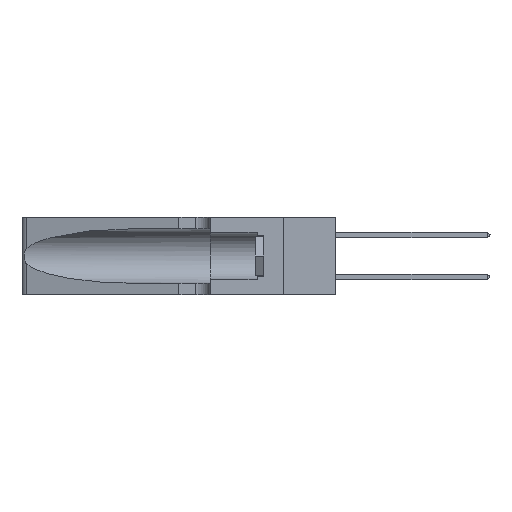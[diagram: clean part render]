
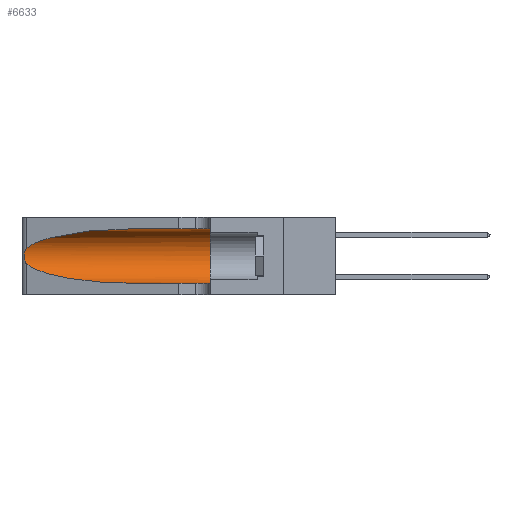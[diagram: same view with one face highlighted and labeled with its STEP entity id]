
A CAD part, left-side view. The second image highlights one B-rep face of the part: STEP entity #6633.
In plain terms, the highlighted cylindrical face has radius 3.308 mm (diameter 6.617 mm), a partial arc.
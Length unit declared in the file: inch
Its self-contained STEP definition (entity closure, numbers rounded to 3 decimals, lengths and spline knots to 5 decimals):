
#329 = CARTESIAN_POINT ( 'NONE',  ( 0.1305, 1.61858, 0.31525 ) ) ;
#985 = CARTESIAN_POINT ( 'NONE',  ( 0.25854, 1.2359, 0.20912 ) ) ;
#3016 = VERTEX_POINT ( 'NONE', #15872 ) ;
#3162 = CARTESIAN_POINT ( 'NONE',  ( 0.25487, 1.22718, 0.22369 ) ) ;
#3678 = DIRECTION ( 'NONE',  ( 0., 1., 0. ) ) ;
#3723 = CARTESIAN_POINT ( 'NONE',  ( 0.26075, 1.23896, 0.19203 ) ) ;
#4461 =( BOUNDED_CURVE ( )  B_SPLINE_CURVE ( 3, ( #12439, #17626, #32968, #30486 ),
 .UNSPECIFIED., .F., .T. ) 
 B_SPLINE_CURVE_WITH_KNOTS ( ( 4, 4 ),
 ( 1.5708, 2.84003 ),
 .UNSPECIFIED. ) 
 CURVE ( )  GEOMETRIC_REPRESENTATION_ITEM ( )  RATIONAL_B_SPLINE_CURVE ( ( 1., 0.87, 0.87, 1. ) ) 
 REPRESENTATION_ITEM ( '' )  );
#5257 = CYLINDRICAL_SURFACE ( 'NONE', #20227, 0.13025 ) ;
#6400 = CARTESIAN_POINT ( 'NONE',  ( 0.26017, 1.23833, 0.17102 ) ) ;
#6633 = ADVANCED_FACE ( 'NONE', ( #32907 ), #5257, .F. ) ;
#7855 = ORIENTED_EDGE ( 'NONE', *, *, #28544, .F. ) ;
#8418 = DIRECTION ( 'NONE',  ( 0., -1., 0. ) ) ;
#8739 = VECTOR ( 'NONE', #8418, 39.37008 ) ;
#9041 = CIRCLE ( 'NONE', #21484, 0.13025 ) ;
#9080 = CARTESIAN_POINT ( 'NONE',  ( 0.25789, 1.23486, 0.15765 ) ) ;
#9450 = CARTESIAN_POINT ( 'NONE',  ( 0.25487, 1.22718, 0.14631 ) ) ;
#10748 = EDGE_CURVE ( 'NONE', #20262, #17674, #4461, .T. ) ;
#11641 = CARTESIAN_POINT ( 'NONE',  ( 0.25487, 1.22718, 0.22369 ) ) ;
#11649 = LINE ( 'NONE', #12639, #25472 ) ;
#11751 = CARTESIAN_POINT ( 'NONE',  ( 0.25555, 1.22993, 0.14849 ) ) ;
#12037 = EDGE_CURVE ( 'NONE', #17674, #29890, #26266, .T. ) ;
#12387 = ORIENTED_EDGE ( 'NONE', *, *, #22652, .T. ) ;
#12439 = CARTESIAN_POINT ( 'NONE',  ( 0.1305, 0.72297, 0.31525 ) ) ;
#12639 = CARTESIAN_POINT ( 'NONE',  ( 0.1305, 1.61858, 0.05475 ) ) ;
#12677 = CARTESIAN_POINT ( 'NONE',  ( 0.1305, 0.72297, 0.05475 ) ) ;
#13414 = CARTESIAN_POINT ( 'NONE',  ( 0.1305, 0.35, 0.31525 ) ) ;
#13920 = ORIENTED_EDGE ( 'NONE', *, *, #27104, .F. ) ;
#14134 = CARTESIAN_POINT ( 'NONE',  ( 0.1305, 0.72297, 0.31525 ) ) ;
#14253 = ORIENTED_EDGE ( 'NONE', *, *, #12037, .T. ) ;
#15003 = VERTEX_POINT ( 'NONE', #13414 ) ;
#15872 = CARTESIAN_POINT ( 'NONE',  ( 0.1305, 0.35, 0.05475 ) ) ;
#16059 = CARTESIAN_POINT ( 'NONE',  ( 0.1305, 0.72297, 0.05475 ) ) ;
#16940 = CARTESIAN_POINT ( 'NONE',  ( 0.25787, 1.23484, 0.2124 ) ) ;
#17626 = CARTESIAN_POINT ( 'NONE',  ( 0.18966, 0.96281, 0.31525 ) ) ;
#17674 = VERTEX_POINT ( 'NONE', #3162 ) ;
#19488 = CARTESIAN_POINT ( 'NONE',  ( 0.1305, 0.35, 0.185 ) ) ;
#19534 = CARTESIAN_POINT ( 'NONE',  ( 0.26018, 1.23835, 0.19895 ) ) ;
#20227 = AXIS2_PLACEMENT_3D ( 'NONE', #25670, #30798, #23133 ) ;
#20262 = VERTEX_POINT ( 'NONE', #14134 ) ;
#20458 = CARTESIAN_POINT ( 'NONE',  ( 0.2373, 1.15595, 0.08982 ) ) ;
#21456 = VERTEX_POINT ( 'NONE', #16059 ) ;
#21484 = AXIS2_PLACEMENT_3D ( 'NONE', #19488, #3678, #22094 ) ;
#21751 = EDGE_LOOP ( 'NONE', ( #27761, #14253, #21763, #12387, #7855, #13920 ) ) ;
#21763 = ORIENTED_EDGE ( 'NONE', *, *, #21977, .T. ) ;
#21977 = EDGE_CURVE ( 'NONE', #29890, #21456, #29722, .T. ) ;
#22094 = DIRECTION ( 'NONE',  ( 0., 0., 1. ) ) ;
#22138 = CARTESIAN_POINT ( 'NONE',  ( 0.26075, 1.23896, 0.178 ) ) ;
#22652 = EDGE_CURVE ( 'NONE', #21456, #3016, #11649, .T. ) ;
#23133 = DIRECTION ( 'NONE',  ( 0., 0., -1. ) ) ;
#24708 = CARTESIAN_POINT ( 'NONE',  ( 0.25856, 1.23593, 0.16098 ) ) ;
#25472 = VECTOR ( 'NONE', #30699, 39.37008 ) ;
#25617 = CARTESIAN_POINT ( 'NONE',  ( 0.25487, 1.22718, 0.14631 ) ) ;
#25670 = CARTESIAN_POINT ( 'NONE',  ( 0.1305, 1.61858, 0.185 ) ) ;
#26266 = B_SPLINE_CURVE_WITH_KNOTS ( 'NONE', 3,
 ( #11641, #29718, #32287, #16940, #985, #19534, #3723, #22138, #6400, #24708, #9080, #27280, #11751, #29837 ),
 .UNSPECIFIED., .F., .F.,
 ( 4, 2, 2, 2, 2, 2, 4 ),
 ( 0., 0.00027, 0.00053, 0.00107, 0.0016, 0.00187, 0.00214 ),
 .UNSPECIFIED. ) ;
#27104 = EDGE_CURVE ( 'NONE', #20262, #15003, #29453, .T. ) ;
#27280 = CARTESIAN_POINT ( 'NONE',  ( 0.25639, 1.23186, 0.15144 ) ) ;
#27761 = ORIENTED_EDGE ( 'NONE', *, *, #10748, .T. ) ;
#28200 = CARTESIAN_POINT ( 'NONE',  ( 0.18966, 0.96281, 0.05475 ) ) ;
#28544 = EDGE_CURVE ( 'NONE', #15003, #3016, #9041, .T. ) ;
#29453 = LINE ( 'NONE', #329, #8739 ) ;
#29718 = CARTESIAN_POINT ( 'NONE',  ( 0.25555, 1.22994, 0.2215 ) ) ;
#29722 =( BOUNDED_CURVE ( )  B_SPLINE_CURVE ( 3, ( #25617, #20458, #28200, #12677 ),
 .UNSPECIFIED., .F., .T. ) 
 B_SPLINE_CURVE_WITH_KNOTS ( ( 4, 4 ),
 ( 3.44316, 4.71239 ),
 .UNSPECIFIED. ) 
 CURVE ( )  GEOMETRIC_REPRESENTATION_ITEM ( )  RATIONAL_B_SPLINE_CURVE ( ( 1., 0.87, 0.87, 1. ) ) 
 REPRESENTATION_ITEM ( '' )  );
#29837 = CARTESIAN_POINT ( 'NONE',  ( 0.25487, 1.22718, 0.14631 ) ) ;
#29890 = VERTEX_POINT ( 'NONE', #9450 ) ;
#30486 = CARTESIAN_POINT ( 'NONE',  ( 0.25487, 1.22718, 0.22369 ) ) ;
#30699 = DIRECTION ( 'NONE',  ( 0., -1., 0. ) ) ;
#30798 = DIRECTION ( 'NONE',  ( 0., -1., 0. ) ) ;
#32287 = CARTESIAN_POINT ( 'NONE',  ( 0.25639, 1.23184, 0.21858 ) ) ;
#32907 = FACE_OUTER_BOUND ( 'NONE', #21751, .T. ) ;
#32968 = CARTESIAN_POINT ( 'NONE',  ( 0.2373, 1.15595, 0.28018 ) ) ;
